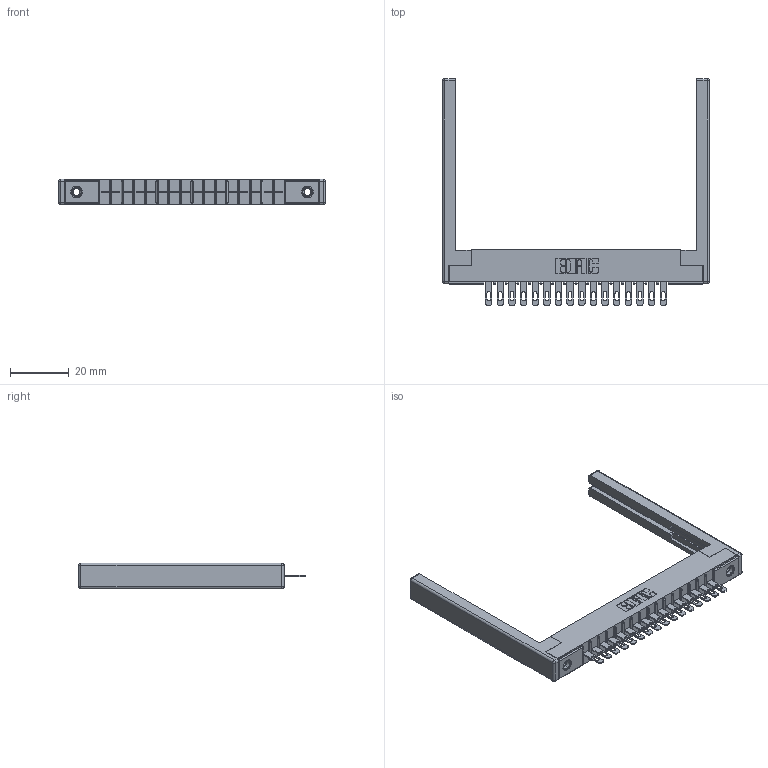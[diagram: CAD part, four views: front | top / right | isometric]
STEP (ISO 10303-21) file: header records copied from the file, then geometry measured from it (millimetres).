
FILE_DESCRIPTION (( 'STEP AP203' ), '1' );
FILE_NAME ('356-016-500-168.STEP', '2018-08-01T19:15:42', ( '' ), ( '' ), 'SwSTEP 2.0', 'SolidWorks 2016', '' );
FILE_SCHEMA (( 'CONFIG_CONTROL_DESIGN' ));
Length unit declared in the file: inch
Products named in the file (5): 306 Part_.156 Dia; 306-290-001_100; 345-250-001_345-250-001-102; 307-220-068; 356-016-500-168
Assembly tree (21 placements, depth 2):
  356-016-500-168
    306 Part_.156 Dia
    306-290-001_100  x16
    345-250-001_345-250-001-102  x2
    307-220-068  x2
Bounding box: 90.83 x 77.17 x 8.71 mm (x, y, z)
Volume: 10781.4 mm3; surface area: 13403.1 mm2
Topology: 21 solids, 21 shells, 1486 faces, 4146 edges, 2656 vertices
Faces by surface type: plane 956, cylinder 442, sphere 72, cone 12, torus 4
Entity records: 21212 total; most frequent: CARTESIAN_POINT 3524, DIRECTION 3491, ORIENTED_EDGE 3482, EDGE_CURVE 1741, VECTOR 1341, LINE 1341, VERTEX_POINT 1108, AXIS2_PLACEMENT_3D 1075
